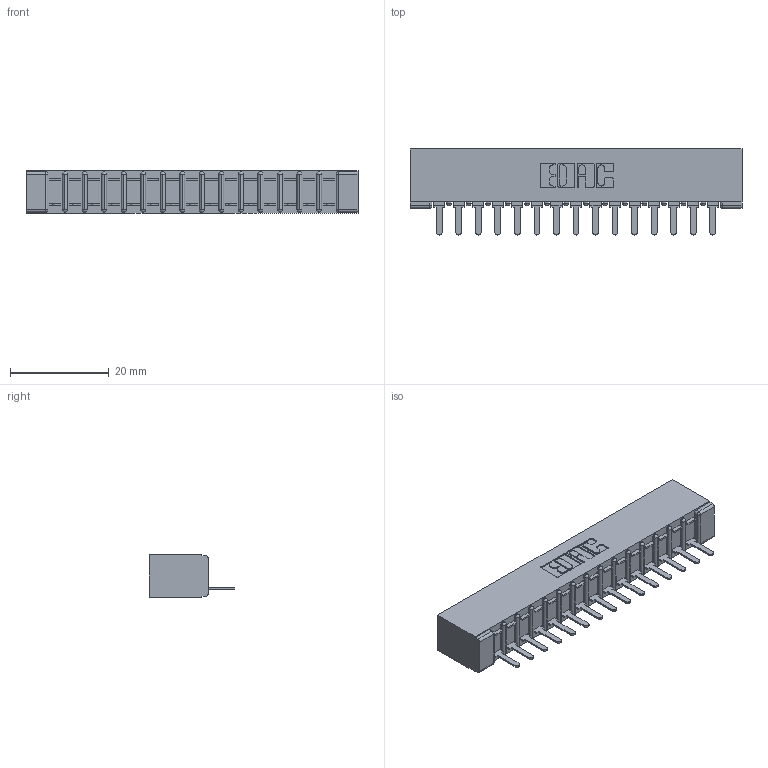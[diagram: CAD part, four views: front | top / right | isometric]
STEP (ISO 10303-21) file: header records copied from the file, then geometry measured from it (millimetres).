
FILE_DESCRIPTION (( 'STEP AP203' ), '1' );
FILE_NAME ('357-015-521-101.STEP', '2018-08-08T01:18:10', ( '' ), ( '' ), 'SwSTEP 2.0', 'SolidWorks 2016', '' );
FILE_SCHEMA (( 'CONFIG_CONTROL_DESIGN' ));
Length unit declared in the file: inch
Products named in the file (3): 307 Part_No Mounting Lugs; 307-290-002_521; 357-015-521-101
Assembly tree (16 placements, depth 2):
  357-015-521-101
    307 Part_No Mounting Lugs
    307-290-002_521  x15
Bounding box: 67.31 x 17.42 x 8.71 mm (x, y, z)
Volume: 4683.2 mm3; surface area: 8644.9 mm2
Topology: 16 solids, 16 shells, 1236 faces, 3779 edges, 2474 vertices
Faces by surface type: plane 741, cylinder 463, sphere 32
Entity records: 16628 total; most frequent: CARTESIAN_POINT 2800, ORIENTED_EDGE 2790, DIRECTION 2731, EDGE_CURVE 1395, VECTOR 1057, LINE 1057, VERTEX_POINT 906, AXIS2_PLACEMENT_3D 837
